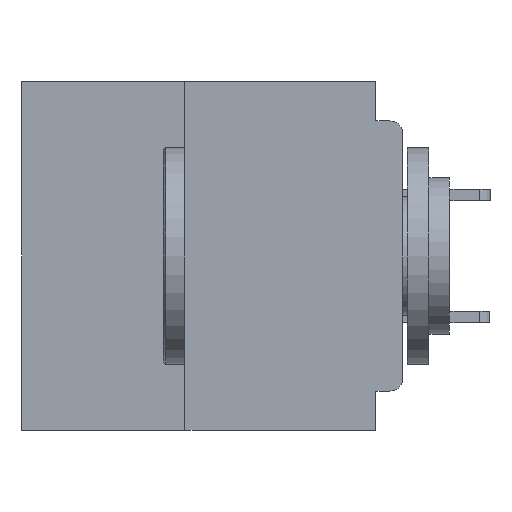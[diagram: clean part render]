
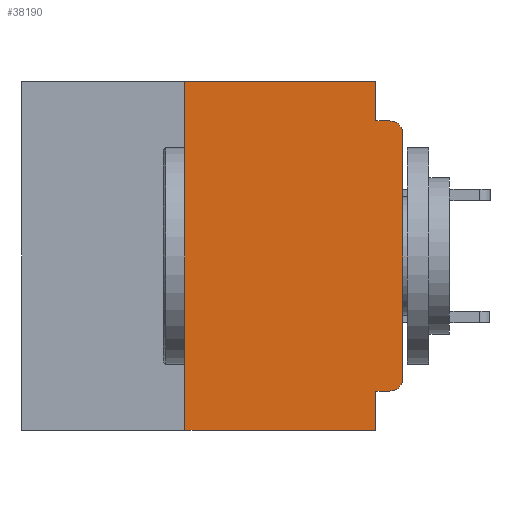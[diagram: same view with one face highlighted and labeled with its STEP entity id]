
A CAD part, left-side view. The second image highlights one B-rep face of the part: STEP entity #38190.
In plain terms, the highlighted planar face has unit normal (-1, 0, 0).
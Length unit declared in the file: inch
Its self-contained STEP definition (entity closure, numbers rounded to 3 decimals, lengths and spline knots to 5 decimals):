
#746 = ORIENTED_EDGE ( 'NONE', *, *, #16765, .T. ) ;
#1088 = VERTEX_POINT ( 'NONE', #47552 ) ;
#2815 = CARTESIAN_POINT ( 'NONE',  ( 0., 0.015, -0.045 ) ) ;
#4161 = ORIENTED_EDGE ( 'NONE', *, *, #15674, .T. ) ;
#4202 = VERTEX_POINT ( 'NONE', #22176 ) ;
#4546 = CARTESIAN_POINT ( 'NONE',  ( 0., 0.031, -0.045 ) ) ;
#4782 = LINE ( 'NONE', #9741, #50412 ) ;
#5244 = VERTEX_POINT ( 'NONE', #24990 ) ;
#5775 = DIRECTION ( 'NONE',  ( -1., 0., 0. ) ) ;
#6958 = CIRCLE ( 'NONE', #45152, 0.015 ) ;
#7918 = LINE ( 'NONE', #52517, #30155 ) ;
#8813 = VECTOR ( 'NONE', #45749, 39.37008 ) ;
#9741 = CARTESIAN_POINT ( 'NONE',  ( 0., 0., -0.355 ) ) ;
#10051 = CARTESIAN_POINT ( 'NONE',  ( 0., 0.25, -0.4 ) ) ;
#10413 = CARTESIAN_POINT ( 'NONE',  ( 0., 0.031, -0.4 ) ) ;
#11884 = ORIENTED_EDGE ( 'NONE', *, *, #52206, .F. ) ;
#13440 = FACE_OUTER_BOUND ( 'NONE', #21246, .T. ) ;
#13691 = CARTESIAN_POINT ( 'NONE',  ( 0., 0.015, -0.355 ) ) ;
#14185 = LINE ( 'NONE', #27373, #48004 ) ;
#14738 = CARTESIAN_POINT ( 'NONE',  ( 0., 0.437, 0. ) ) ;
#14868 = CARTESIAN_POINT ( 'NONE',  ( 0., 0.25, -0.4 ) ) ;
#15027 = VERTEX_POINT ( 'NONE', #43384 ) ;
#15674 = EDGE_CURVE ( 'NONE', #4202, #20516, #14185, .T. ) ;
#16356 = EDGE_CURVE ( 'NONE', #15027, #1088, #47584, .T. ) ;
#16765 = EDGE_CURVE ( 'NONE', #20516, #40292, #31061, .T. ) ;
#17878 = DIRECTION ( 'NONE',  ( 0., -1., 0. ) ) ;
#18107 = VERTEX_POINT ( 'NONE', #40220 ) ;
#18641 = DIRECTION ( 'NONE',  ( 0., 0., 1. ) ) ;
#18714 = ORIENTED_EDGE ( 'NONE', *, *, #36120, .F. ) ;
#18799 = VECTOR ( 'NONE', #53371, 39.37008 ) ;
#19199 = DIRECTION ( 'NONE',  ( 0., -1., 0. ) ) ;
#19332 = EDGE_CURVE ( 'NONE', #24960, #1088, #7918, .T. ) ;
#20516 = VERTEX_POINT ( 'NONE', #56252 ) ;
#21246 = EDGE_LOOP ( 'NONE', ( #4161, #746, #11884, #45343, #18714, #42971, #57015, #38333, #28059, #32752 ) ) ;
#22176 = CARTESIAN_POINT ( 'NONE',  ( 0., 0., -0.34 ) ) ;
#22288 = EDGE_CURVE ( 'NONE', #24960, #5244, #33807, .T. ) ;
#22768 = DIRECTION ( 'NONE',  ( -1., 0., 0. ) ) ;
#23130 = DIRECTION ( 'NONE',  ( 0., 1., 0. ) ) ;
#24629 = VECTOR ( 'NONE', #17878, 39.37008 ) ;
#24960 = VERTEX_POINT ( 'NONE', #10051 ) ;
#24990 = CARTESIAN_POINT ( 'NONE',  ( 0., 0.25, 0. ) ) ;
#27373 = CARTESIAN_POINT ( 'NONE',  ( 0., 0., 0. ) ) ;
#28059 = ORIENTED_EDGE ( 'NONE', *, *, #31653, .F. ) ;
#28872 = DIRECTION ( 'NONE',  ( 0., 0., -1. ) ) ;
#30155 = VECTOR ( 'NONE', #39338, 39.37008 ) ;
#30606 = LINE ( 'NONE', #48993, #18799 ) ;
#31061 = CIRCLE ( 'NONE', #57086, 0.015 ) ;
#31653 = EDGE_CURVE ( 'NONE', #42984, #15027, #4782, .T. ) ;
#32373 = CARTESIAN_POINT ( 'NONE',  ( 0., 0.015, -0.34 ) ) ;
#32752 = ORIENTED_EDGE ( 'NONE', *, *, #56254, .T. ) ;
#32780 = VERTEX_POINT ( 'NONE', #4546 ) ;
#33114 = CARTESIAN_POINT ( 'NONE',  ( 0., 0.437, 0. ) ) ;
#33807 = LINE ( 'NONE', #14868, #8813 ) ;
#35244 = VECTOR ( 'NONE', #19199, 39.37008 ) ;
#35907 = VECTOR ( 'NONE', #45744, 39.37008 ) ;
#36120 = EDGE_CURVE ( 'NONE', #5244, #18107, #44154, .T. ) ;
#36786 = DIRECTION ( 'NONE',  ( 0., 0., -1. ) ) ;
#38190 = ADVANCED_FACE ( 'NONE', ( #13440 ), #50766, .F. ) ;
#38333 = ORIENTED_EDGE ( 'NONE', *, *, #16356, .F. ) ;
#39338 = DIRECTION ( 'NONE',  ( 0., -1., 0. ) ) ;
#40097 = CARTESIAN_POINT ( 'NONE',  ( 0., 0., -0.045 ) ) ;
#40220 = CARTESIAN_POINT ( 'NONE',  ( 0., 0.031, 0. ) ) ;
#40292 = VERTEX_POINT ( 'NONE', #2815 ) ;
#42971 = ORIENTED_EDGE ( 'NONE', *, *, #22288, .F. ) ;
#42984 = VERTEX_POINT ( 'NONE', #13691 ) ;
#42987 = EDGE_CURVE ( 'NONE', #18107, #32780, #30606, .T. ) ;
#43384 = CARTESIAN_POINT ( 'NONE',  ( 0., 0.031, -0.355 ) ) ;
#44154 = LINE ( 'NONE', #14738, #35244 ) ;
#45152 = AXIS2_PLACEMENT_3D ( 'NONE', #32373, #5775, #36786 ) ;
#45343 = ORIENTED_EDGE ( 'NONE', *, *, #42987, .F. ) ;
#45744 = DIRECTION ( 'NONE',  ( 0., 0., -1. ) ) ;
#45749 = DIRECTION ( 'NONE',  ( 0., 0., 1. ) ) ;
#47552 = CARTESIAN_POINT ( 'NONE',  ( 0., 0.031, -0.4 ) ) ;
#47584 = LINE ( 'NONE', #10413, #35907 ) ;
#48004 = VECTOR ( 'NONE', #18641, 39.37008 ) ;
#48029 = LINE ( 'NONE', #40097, #24629 ) ;
#48993 = CARTESIAN_POINT ( 'NONE',  ( 0., 0.031, 0. ) ) ;
#49165 = CARTESIAN_POINT ( 'NONE',  ( 0., 0.015, -0.06 ) ) ;
#50412 = VECTOR ( 'NONE', #23130, 39.37008 ) ;
#50766 = PLANE ( 'NONE',  #54399 ) ;
#52206 = EDGE_CURVE ( 'NONE', #32780, #40292, #48029, .T. ) ;
#52517 = CARTESIAN_POINT ( 'NONE',  ( 0., 0.437, -0.4 ) ) ;
#53371 = DIRECTION ( 'NONE',  ( 0., 0., -1. ) ) ;
#53558 = DIRECTION ( 'NONE',  ( 0., 0., -1. ) ) ;
#54399 = AXIS2_PLACEMENT_3D ( 'NONE', #33114, #55171, #28872 ) ;
#55171 = DIRECTION ( 'NONE',  ( 1., 0., 0. ) ) ;
#56252 = CARTESIAN_POINT ( 'NONE',  ( 0., 0., -0.06 ) ) ;
#56254 = EDGE_CURVE ( 'NONE', #42984, #4202, #6958, .T. ) ;
#57015 = ORIENTED_EDGE ( 'NONE', *, *, #19332, .T. ) ;
#57086 = AXIS2_PLACEMENT_3D ( 'NONE', #49165, #22768, #53558 ) ;
